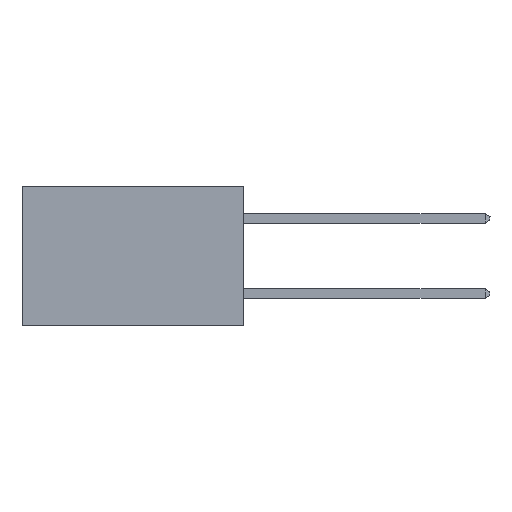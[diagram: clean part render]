
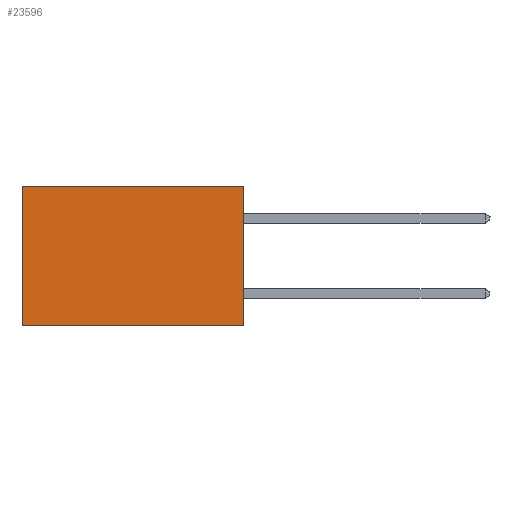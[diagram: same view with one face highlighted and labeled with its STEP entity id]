
A CAD part, left-side view. The second image highlights one B-rep face of the part: STEP entity #23596.
In plain terms, the highlighted planar face has unit normal (-1, 0, 0).
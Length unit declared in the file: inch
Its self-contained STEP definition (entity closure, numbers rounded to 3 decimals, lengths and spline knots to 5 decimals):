
#127 = LINE ( 'NONE', #14165, #15283 ) ;
#176 = DIRECTION ( 'NONE',  ( 0., 0., -1. ) ) ;
#457 = EDGE_CURVE ( 'NONE', #12795, #17132, #8941, .T. ) ;
#3018 = LINE ( 'NONE', #14063, #23022 ) ;
#3911 = CARTESIAN_POINT ( 'NONE',  ( 0.277, 0.59, -0.37 ) ) ;
#4570 = EDGE_LOOP ( 'NONE', ( #17389, #24208, #13685, #11469 ) ) ;
#5225 = DIRECTION ( 'NONE',  ( 0., 0., -1. ) ) ;
#7103 = FACE_OUTER_BOUND ( 'NONE', #4570, .T. ) ;
#8793 = VERTEX_POINT ( 'NONE', #13808 ) ;
#8941 = LINE ( 'NONE', #20366, #18592 ) ;
#10782 = EDGE_CURVE ( 'NONE', #17132, #11997, #3018, .T. ) ;
#11346 = CARTESIAN_POINT ( 'NONE',  ( 0.277, 0., -0.37 ) ) ;
#11456 = VECTOR ( 'NONE', #13302, 39.37008 ) ;
#11469 = ORIENTED_EDGE ( 'NONE', *, *, #457, .T. ) ;
#11997 = VERTEX_POINT ( 'NONE', #3911 ) ;
#12795 = VERTEX_POINT ( 'NONE', #24255 ) ;
#13081 = PLANE ( 'NONE',  #15186 ) ;
#13302 = DIRECTION ( 'NONE',  ( 0., 1., 0. ) ) ;
#13685 = ORIENTED_EDGE ( 'NONE', *, *, #21939, .F. ) ;
#13808 = CARTESIAN_POINT ( 'NONE',  ( 0.277, 0., -0.37 ) ) ;
#14063 = CARTESIAN_POINT ( 'NONE',  ( 0.277, 0.59, -0.37 ) ) ;
#14165 = CARTESIAN_POINT ( 'NONE',  ( 0.277, 0., -0.37 ) ) ;
#15016 = CARTESIAN_POINT ( 'NONE',  ( 0.277, 0., -0.37 ) ) ;
#15186 = AXIS2_PLACEMENT_3D ( 'NONE', #15016, #16923, #5225 ) ;
#15283 = VECTOR ( 'NONE', #16087, 39.37008 ) ;
#16087 = DIRECTION ( 'NONE',  ( 0., 0., -1. ) ) ;
#16637 = DIRECTION ( 'NONE',  ( 0., 1., 0. ) ) ;
#16923 = DIRECTION ( 'NONE',  ( 1., 0., 0. ) ) ;
#17132 = VERTEX_POINT ( 'NONE', #24029 ) ;
#17389 = ORIENTED_EDGE ( 'NONE', *, *, #10782, .T. ) ;
#18592 = VECTOR ( 'NONE', #16637, 39.37008 ) ;
#20139 = EDGE_CURVE ( 'NONE', #8793, #11997, #21609, .T. ) ;
#20366 = CARTESIAN_POINT ( 'NONE',  ( 0.277, 0., 0. ) ) ;
#21609 = LINE ( 'NONE', #11346, #11456 ) ;
#21939 = EDGE_CURVE ( 'NONE', #12795, #8793, #127, .T. ) ;
#23022 = VECTOR ( 'NONE', #176, 39.37008 ) ;
#23596 = ADVANCED_FACE ( 'NONE', ( #7103 ), #13081, .F. ) ;
#24029 = CARTESIAN_POINT ( 'NONE',  ( 0.277, 0.59, 0. ) ) ;
#24208 = ORIENTED_EDGE ( 'NONE', *, *, #20139, .F. ) ;
#24255 = CARTESIAN_POINT ( 'NONE',  ( 0.277, 0., 0. ) ) ;
